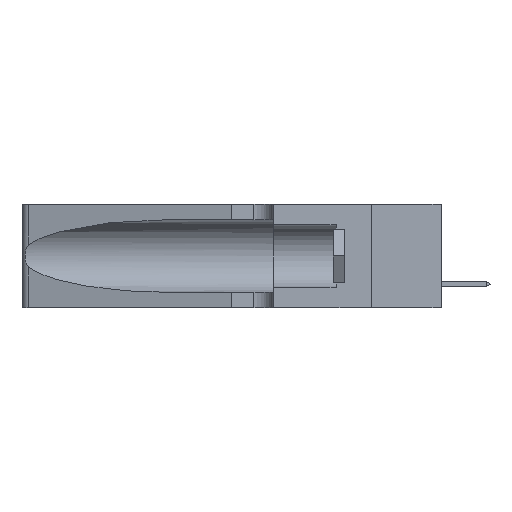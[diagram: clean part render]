
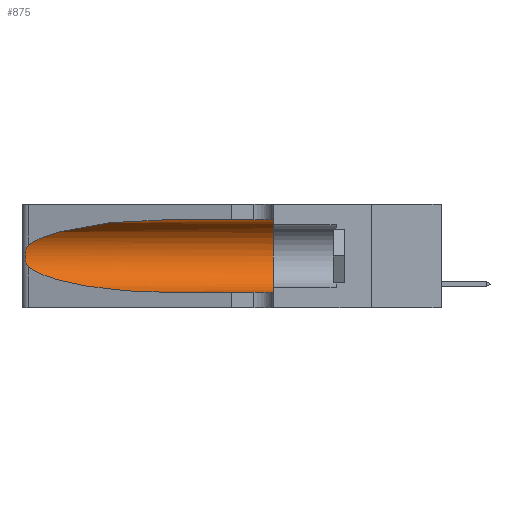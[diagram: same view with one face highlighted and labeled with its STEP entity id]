
A CAD part, left-side view. The second image highlights one B-rep face of the part: STEP entity #875.
In plain terms, the highlighted cylindrical face has radius 3.308 mm (diameter 6.617 mm), a partial arc.
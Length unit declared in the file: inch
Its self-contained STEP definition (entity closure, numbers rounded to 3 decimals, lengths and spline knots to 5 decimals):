
#538 = CARTESIAN_POINT ( 'NONE',  ( 0.1305, 0.72297, 0.31525 ) ) ;
#617 = CARTESIAN_POINT ( 'NONE',  ( 0.18966, 0.96281, 0.05475 ) ) ;
#875 = ADVANCED_FACE ( 'NONE', ( #5584 ), #51869, .F. ) ;
#1415 = AXIS2_PLACEMENT_3D ( 'NONE', #28428, #12534, #4582 ) ;
#1659 = CARTESIAN_POINT ( 'NONE',  ( 0.25789, 1.23486, 0.15765 ) ) ;
#2285 = B_SPLINE_CURVE_WITH_KNOTS ( 'NONE', 3,
 ( #45957, #9678, #10037, #30166, #37984, #29781, #21983, #34098, #50188, #5605, #1659, #29976, #33916, #13191 ),
 .UNSPECIFIED., .F., .F.,
 ( 4, 2, 2, 2, 2, 2, 4 ),
 ( 0., 0.00027, 0.00053, 0.00107, 0.0016, 0.00187, 0.00214 ),
 .UNSPECIFIED. ) ;
#3314 = EDGE_LOOP ( 'NONE', ( #32049, #26030, #19416, #22363, #26512, #12814 ) ) ;
#3664 = CARTESIAN_POINT ( 'NONE',  ( 0.2373, 1.15595, 0.28018 ) ) ;
#4582 = DIRECTION ( 'NONE',  ( 0., 0., 1. ) ) ;
#4614 = CARTESIAN_POINT ( 'NONE',  ( 0.25487, 1.22718, 0.14631 ) ) ;
#5584 = FACE_OUTER_BOUND ( 'NONE', #3314, .T. ) ;
#5605 = CARTESIAN_POINT ( 'NONE',  ( 0.25856, 1.23593, 0.16098 ) ) ;
#7345 = CARTESIAN_POINT ( 'NONE',  ( 0.1305, 0.35, 0.31525 ) ) ;
#8338 = EDGE_CURVE ( 'NONE', #31876, #36014, #21516, .T. ) ;
#9516 = CARTESIAN_POINT ( 'NONE',  ( 0.1305, 0.72297, 0.05475 ) ) ;
#9678 = CARTESIAN_POINT ( 'NONE',  ( 0.25555, 1.22994, 0.2215 ) ) ;
#10037 = CARTESIAN_POINT ( 'NONE',  ( 0.25639, 1.23184, 0.21858 ) ) ;
#10820 = VERTEX_POINT ( 'NONE', #9516 ) ;
#12532 = CARTESIAN_POINT ( 'NONE',  ( 0.25487, 1.22718, 0.14631 ) ) ;
#12534 = DIRECTION ( 'NONE',  ( 0., 1., 0. ) ) ;
#12814 = ORIENTED_EDGE ( 'NONE', *, *, #8338, .F. ) ;
#12953 = CARTESIAN_POINT ( 'NONE',  ( 0.25487, 1.22718, 0.22369 ) ) ;
#13191 = CARTESIAN_POINT ( 'NONE',  ( 0.25487, 1.22718, 0.14631 ) ) ;
#13644 = VERTEX_POINT ( 'NONE', #4614 ) ;
#15674 = CARTESIAN_POINT ( 'NONE',  ( 0.1305, 1.61858, 0.31525 ) ) ;
#15975 = EDGE_CURVE ( 'NONE', #36014, #28753, #38941, .T. ) ;
#16894 = EDGE_CURVE ( 'NONE', #45716, #13644, #2285, .T. ) ;
#19154 = VECTOR ( 'NONE', #43468, 39.37008 ) ;
#19416 = ORIENTED_EDGE ( 'NONE', *, *, #33345, .T. ) ;
#21516 = LINE ( 'NONE', #15674, #26666 ) ;
#21983 = CARTESIAN_POINT ( 'NONE',  ( 0.26075, 1.23896, 0.19203 ) ) ;
#22363 = ORIENTED_EDGE ( 'NONE', *, *, #24134, .T. ) ;
#24134 = EDGE_CURVE ( 'NONE', #10820, #28753, #29810, .T. ) ;
#26030 = ORIENTED_EDGE ( 'NONE', *, *, #16894, .T. ) ;
#26512 = ORIENTED_EDGE ( 'NONE', *, *, #15975, .F. ) ;
#26602 = DIRECTION ( 'NONE',  ( 0., 0., -1. ) ) ;
#26666 = VECTOR ( 'NONE', #39411, 39.37008 ) ;
#28428 = CARTESIAN_POINT ( 'NONE',  ( 0.1305, 0.35, 0.185 ) ) ;
#28753 = VERTEX_POINT ( 'NONE', #41917 ) ;
#29781 = CARTESIAN_POINT ( 'NONE',  ( 0.26018, 1.23835, 0.19895 ) ) ;
#29810 = LINE ( 'NONE', #39216, #19154 ) ;
#29976 = CARTESIAN_POINT ( 'NONE',  ( 0.25639, 1.23186, 0.15144 ) ) ;
#30166 = CARTESIAN_POINT ( 'NONE',  ( 0.25787, 1.23484, 0.2124 ) ) ;
#31876 = VERTEX_POINT ( 'NONE', #42127 ) ;
#32049 = ORIENTED_EDGE ( 'NONE', *, *, #45069, .T. ) ;
#32888 = CARTESIAN_POINT ( 'NONE',  ( 0.2373, 1.15595, 0.08982 ) ) ;
#33345 = EDGE_CURVE ( 'NONE', #13644, #10820, #37635, .T. ) ;
#33916 = CARTESIAN_POINT ( 'NONE',  ( 0.25555, 1.22993, 0.14849 ) ) ;
#34098 = CARTESIAN_POINT ( 'NONE',  ( 0.26075, 1.23896, 0.178 ) ) ;
#34295 = AXIS2_PLACEMENT_3D ( 'NONE', #42609, #50516, #26602 ) ;
#36014 = VERTEX_POINT ( 'NONE', #7345 ) ;
#37635 =( BOUNDED_CURVE ( )  B_SPLINE_CURVE ( 3, ( #12532, #32888, #617, #38560 ),
 .UNSPECIFIED., .F., .F. ) 
 B_SPLINE_CURVE_WITH_KNOTS ( ( 4, 4 ),
 ( 3.44316, 4.71239 ),
 .UNSPECIFIED. ) 
 CURVE ( )  GEOMETRIC_REPRESENTATION_ITEM ( )  RATIONAL_B_SPLINE_CURVE ( ( 1., 0.87, 0.87, 1. ) ) 
 REPRESENTATION_ITEM ( '' )  );
#37984 = CARTESIAN_POINT ( 'NONE',  ( 0.25854, 1.2359, 0.20912 ) ) ;
#38560 = CARTESIAN_POINT ( 'NONE',  ( 0.1305, 0.72297, 0.05475 ) ) ;
#38941 = CIRCLE ( 'NONE', #1415, 0.13025 ) ;
#39216 = CARTESIAN_POINT ( 'NONE',  ( 0.1305, 1.61858, 0.05475 ) ) ;
#39411 = DIRECTION ( 'NONE',  ( 0., -1., 0. ) ) ;
#41917 = CARTESIAN_POINT ( 'NONE',  ( 0.1305, 0.35, 0.05475 ) ) ;
#42127 = CARTESIAN_POINT ( 'NONE',  ( 0.1305, 0.72297, 0.31525 ) ) ;
#42609 = CARTESIAN_POINT ( 'NONE',  ( 0.1305, 1.61858, 0.185 ) ) ;
#43468 = DIRECTION ( 'NONE',  ( 0., -1., 0. ) ) ;
#45069 = EDGE_CURVE ( 'NONE', #31876, #45716, #45448, .T. ) ;
#45202 = CARTESIAN_POINT ( 'NONE',  ( 0.18966, 0.96281, 0.31525 ) ) ;
#45448 =( BOUNDED_CURVE ( )  B_SPLINE_CURVE ( 3, ( #538, #45202, #3664, #12953 ),
 .UNSPECIFIED., .F., .F. ) 
 B_SPLINE_CURVE_WITH_KNOTS ( ( 4, 4 ),
 ( 1.5708, 2.84003 ),
 .UNSPECIFIED. ) 
 CURVE ( )  GEOMETRIC_REPRESENTATION_ITEM ( )  RATIONAL_B_SPLINE_CURVE ( ( 1., 0.87, 0.87, 1. ) ) 
 REPRESENTATION_ITEM ( '' )  );
#45716 = VERTEX_POINT ( 'NONE', #51026 ) ;
#45957 = CARTESIAN_POINT ( 'NONE',  ( 0.25487, 1.22718, 0.22369 ) ) ;
#50188 = CARTESIAN_POINT ( 'NONE',  ( 0.26017, 1.23833, 0.17102 ) ) ;
#50516 = DIRECTION ( 'NONE',  ( 0., -1., 0. ) ) ;
#51026 = CARTESIAN_POINT ( 'NONE',  ( 0.25487, 1.22718, 0.22369 ) ) ;
#51869 = CYLINDRICAL_SURFACE ( 'NONE', #34295, 0.13025 ) ;
